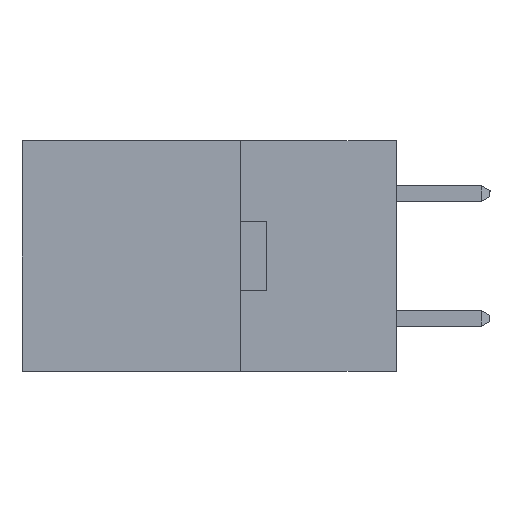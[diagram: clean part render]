
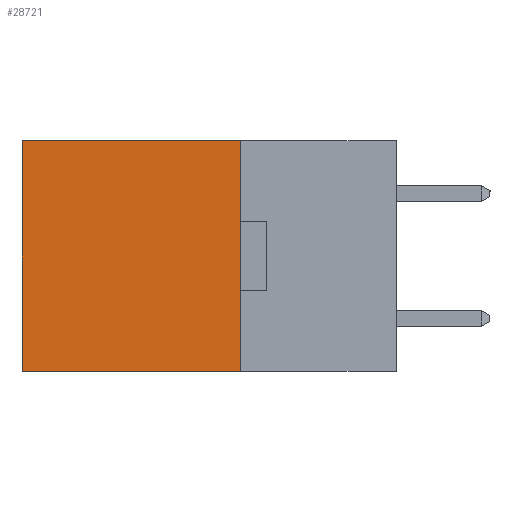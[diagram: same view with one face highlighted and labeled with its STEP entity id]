
A CAD part, left-side view. The second image highlights one B-rep face of the part: STEP entity #28721.
In plain terms, the highlighted planar face has unit normal (-1, 0, 0).
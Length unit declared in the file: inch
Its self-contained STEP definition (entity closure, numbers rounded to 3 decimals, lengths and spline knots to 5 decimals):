
#2431 = LINE ( 'NONE', #6488, #22438 ) ;
#2472 = LINE ( 'NONE', #7401, #12294 ) ;
#3460 = CARTESIAN_POINT ( 'NONE',  ( 0.2615, 0.25, 0. ) ) ;
#5000 = CARTESIAN_POINT ( 'NONE',  ( 0.2615, 0.6, 0. ) ) ;
#6488 = CARTESIAN_POINT ( 'NONE',  ( 0.2615, 0.25, -0.37 ) ) ;
#6577 = VECTOR ( 'NONE', #13302, 39.37008 ) ;
#7401 = CARTESIAN_POINT ( 'NONE',  ( 0.2615, 0.25, -0.37 ) ) ;
#7775 = FACE_OUTER_BOUND ( 'NONE', #22650, .T. ) ;
#8102 = ORIENTED_EDGE ( 'NONE', *, *, #11921, .F. ) ;
#8446 = VERTEX_POINT ( 'NONE', #27166 ) ;
#9870 = VERTEX_POINT ( 'NONE', #18886 ) ;
#11762 = VERTEX_POINT ( 'NONE', #3460 ) ;
#11921 = EDGE_CURVE ( 'NONE', #11762, #8446, #2431, .T. ) ;
#12294 = VECTOR ( 'NONE', #17932, 39.37008 ) ;
#13302 = DIRECTION ( 'NONE',  ( 0., 1., 0. ) ) ;
#15055 = LINE ( 'NONE', #19890, #6577 ) ;
#16548 = VECTOR ( 'NONE', #17704, 39.37008 ) ;
#17227 = EDGE_CURVE ( 'NONE', #8446, #9870, #2472, .T. ) ;
#17704 = DIRECTION ( 'NONE',  ( 0., 0., -1. ) ) ;
#17932 = DIRECTION ( 'NONE',  ( 0., 1., 0. ) ) ;
#18003 = EDGE_CURVE ( 'NONE', #20687, #9870, #24242, .T. ) ;
#18114 = ORIENTED_EDGE ( 'NONE', *, *, #17227, .F. ) ;
#18886 = CARTESIAN_POINT ( 'NONE',  ( 0.2615, 0.6, -0.37 ) ) ;
#19017 = DIRECTION ( 'NONE',  ( 0., 0., -1. ) ) ;
#19890 = CARTESIAN_POINT ( 'NONE',  ( 0.2615, 0.25, 0. ) ) ;
#20527 = DIRECTION ( 'NONE',  ( 0., 0., -1. ) ) ;
#20687 = VERTEX_POINT ( 'NONE', #5000 ) ;
#20788 = DIRECTION ( 'NONE',  ( 1., 0., 0. ) ) ;
#22024 = AXIS2_PLACEMENT_3D ( 'NONE', #23232, #20788, #19017 ) ;
#22231 = CARTESIAN_POINT ( 'NONE',  ( 0.2615, 0.6, -0.37 ) ) ;
#22438 = VECTOR ( 'NONE', #20527, 39.37008 ) ;
#22650 = EDGE_LOOP ( 'NONE', ( #27942, #18114, #8102, #24022 ) ) ;
#23232 = CARTESIAN_POINT ( 'NONE',  ( 0.2615, 0.25, -0.37 ) ) ;
#23375 = PLANE ( 'NONE',  #22024 ) ;
#24022 = ORIENTED_EDGE ( 'NONE', *, *, #27393, .T. ) ;
#24242 = LINE ( 'NONE', #22231, #16548 ) ;
#27166 = CARTESIAN_POINT ( 'NONE',  ( 0.2615, 0.25, -0.37 ) ) ;
#27393 = EDGE_CURVE ( 'NONE', #11762, #20687, #15055, .T. ) ;
#27942 = ORIENTED_EDGE ( 'NONE', *, *, #18003, .T. ) ;
#28721 = ADVANCED_FACE ( 'NONE', ( #7775 ), #23375, .F. ) ;
